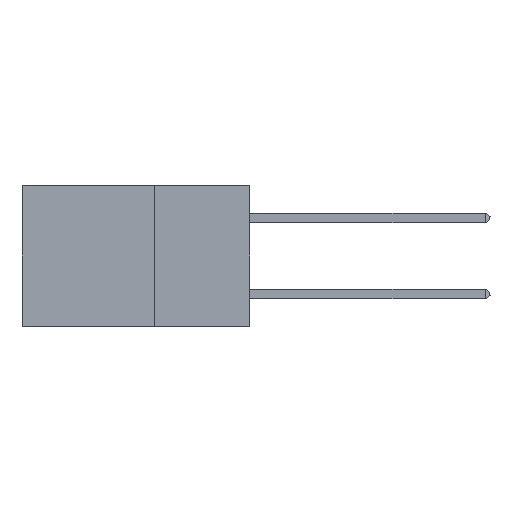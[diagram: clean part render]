
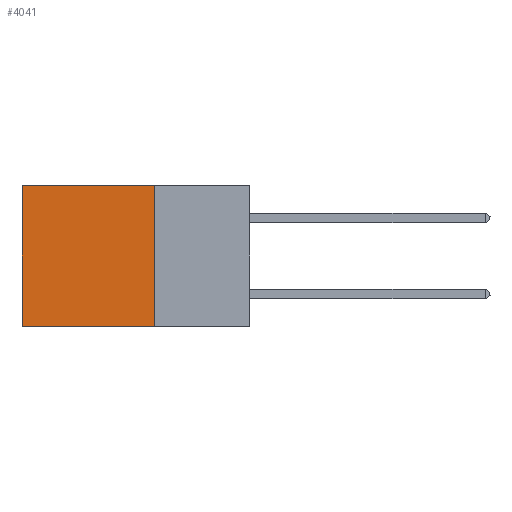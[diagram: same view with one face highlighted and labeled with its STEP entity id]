
A CAD part, left-side view. The second image highlights one B-rep face of the part: STEP entity #4041.
In plain terms, the highlighted planar face has unit normal (-1, 0, 0).
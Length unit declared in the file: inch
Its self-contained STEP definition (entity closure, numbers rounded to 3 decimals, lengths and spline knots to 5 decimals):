
#1419 = EDGE_CURVE ( 'NONE', #24009, #27615, #36870, .T. ) ;
#2310 = LINE ( 'NONE', #42746, #42216 ) ;
#2454 = CARTESIAN_POINT ( 'NONE',  ( 0.2875, 0.25, 0. ) ) ;
#2510 = VERTEX_POINT ( 'NONE', #18118 ) ;
#4041 = ADVANCED_FACE ( 'NONE', ( #17774 ), #29192, .F. ) ;
#4900 = EDGE_CURVE ( 'NONE', #2510, #24009, #36841, .T. ) ;
#5185 = DIRECTION ( 'NONE',  ( 0., 1., 0. ) ) ;
#6169 = DIRECTION ( 'NONE',  ( 0., 0., -1. ) ) ;
#8850 = CARTESIAN_POINT ( 'NONE',  ( 0.2875, 0.25, 0. ) ) ;
#9732 = VECTOR ( 'NONE', #29666, 39.37008 ) ;
#10298 = EDGE_CURVE ( 'NONE', #19487, #27615, #2310, .T. ) ;
#10394 = LINE ( 'NONE', #31635, #18372 ) ;
#11268 = CARTESIAN_POINT ( 'NONE',  ( 0.2875, 0.6, -0.37 ) ) ;
#12316 = EDGE_LOOP ( 'NONE', ( #38800, #22496, #31274, #40321 ) ) ;
#12873 = DIRECTION ( 'NONE',  ( 1., 0., 0. ) ) ;
#14847 = DIRECTION ( 'NONE',  ( 0., 1., 0. ) ) ;
#17774 = FACE_OUTER_BOUND ( 'NONE', #12316, .T. ) ;
#18118 = CARTESIAN_POINT ( 'NONE',  ( 0.2875, 0.25, 0. ) ) ;
#18372 = VECTOR ( 'NONE', #14847, 39.37008 ) ;
#19487 = VERTEX_POINT ( 'NONE', #37024 ) ;
#22496 = ORIENTED_EDGE ( 'NONE', *, *, #1419, .F. ) ;
#24009 = VERTEX_POINT ( 'NONE', #37815 ) ;
#25557 = CARTESIAN_POINT ( 'NONE',  ( 0.2875, 0.25, -0.37 ) ) ;
#27615 = VERTEX_POINT ( 'NONE', #11268 ) ;
#29090 = DIRECTION ( 'NONE',  ( 0., 0., -1. ) ) ;
#29192 = PLANE ( 'NONE',  #40806 ) ;
#29666 = DIRECTION ( 'NONE',  ( 0., 0., -1. ) ) ;
#31274 = ORIENTED_EDGE ( 'NONE', *, *, #4900, .F. ) ;
#31635 = CARTESIAN_POINT ( 'NONE',  ( 0.2875, 0.25, 0. ) ) ;
#35386 = EDGE_CURVE ( 'NONE', #2510, #19487, #10394, .T. ) ;
#36841 = LINE ( 'NONE', #2454, #9732 ) ;
#36870 = LINE ( 'NONE', #25557, #41106 ) ;
#37024 = CARTESIAN_POINT ( 'NONE',  ( 0.2875, 0.6, 0. ) ) ;
#37815 = CARTESIAN_POINT ( 'NONE',  ( 0.2875, 0.25, -0.37 ) ) ;
#38800 = ORIENTED_EDGE ( 'NONE', *, *, #10298, .T. ) ;
#40321 = ORIENTED_EDGE ( 'NONE', *, *, #35386, .T. ) ;
#40806 = AXIS2_PLACEMENT_3D ( 'NONE', #8850, #12873, #6169 ) ;
#41106 = VECTOR ( 'NONE', #5185, 39.37008 ) ;
#42216 = VECTOR ( 'NONE', #29090, 39.37008 ) ;
#42746 = CARTESIAN_POINT ( 'NONE',  ( 0.2875, 0.6, 0. ) ) ;
